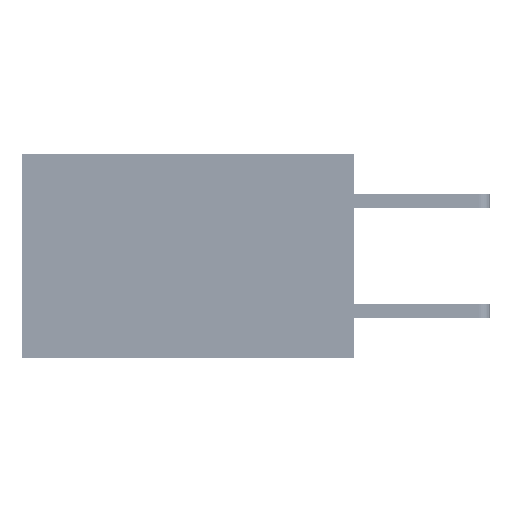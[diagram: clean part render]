
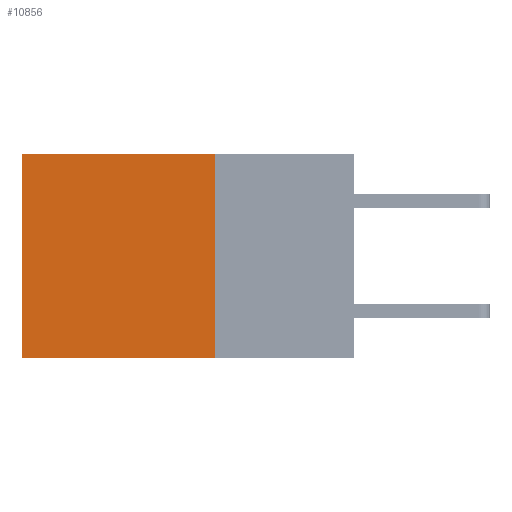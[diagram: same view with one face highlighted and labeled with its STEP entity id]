
A CAD part, left-side view. The second image highlights one B-rep face of the part: STEP entity #10856.
In plain terms, the highlighted planar face has unit normal (-1, 0, 0).
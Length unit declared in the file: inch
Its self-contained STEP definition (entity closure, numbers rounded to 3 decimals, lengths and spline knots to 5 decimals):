
#834 = EDGE_CURVE ( 'NONE', #1383, #25259, #34924, .T. ) ;
#1383 = VERTEX_POINT ( 'NONE', #32622 ) ;
#1986 = DIRECTION ( 'NONE',  ( 0., 1., 0. ) ) ;
#2571 = LINE ( 'NONE', #12450, #19545 ) ;
#5033 = VECTOR ( 'NONE', #1986, 39.37008 ) ;
#5194 = CARTESIAN_POINT ( 'NONE',  ( 0.2875, 0.6, -0.37 ) ) ;
#5345 = DIRECTION ( 'NONE',  ( 1., 0., 0. ) ) ;
#5413 = VERTEX_POINT ( 'NONE', #5194 ) ;
#10572 = EDGE_CURVE ( 'NONE', #1383, #33118, #15360, .T. ) ;
#10856 = ADVANCED_FACE ( 'NONE', ( #25638 ), #35568, .F. ) ;
#12450 = CARTESIAN_POINT ( 'NONE',  ( 0.2875, 0.25, -0.37 ) ) ;
#13830 = ORIENTED_EDGE ( 'NONE', *, *, #36696, .T. ) ;
#14040 = ORIENTED_EDGE ( 'NONE', *, *, #22499, .F. ) ;
#15360 = LINE ( 'NONE', #41514, #5033 ) ;
#18775 = DIRECTION ( 'NONE',  ( 0., 0., -1. ) ) ;
#19130 = CARTESIAN_POINT ( 'NONE',  ( 0.2875, 0.25, 0. ) ) ;
#19545 = VECTOR ( 'NONE', #22377, 39.37008 ) ;
#22377 = DIRECTION ( 'NONE',  ( 0., 1., 0. ) ) ;
#22499 = EDGE_CURVE ( 'NONE', #25259, #5413, #2571, .T. ) ;
#23221 = CARTESIAN_POINT ( 'NONE',  ( 0.2875, 0.25, -0.37 ) ) ;
#23643 = VECTOR ( 'NONE', #18775, 39.37008 ) ;
#24660 = VECTOR ( 'NONE', #38017, 39.37008 ) ;
#25259 = VERTEX_POINT ( 'NONE', #23221 ) ;
#25638 = FACE_OUTER_BOUND ( 'NONE', #25856, .T. ) ;
#25856 = EDGE_LOOP ( 'NONE', ( #13830, #14040, #37893, #31315 ) ) ;
#28336 = CARTESIAN_POINT ( 'NONE',  ( 0.2875, 0.6, 0. ) ) ;
#28402 = DIRECTION ( 'NONE',  ( 0., 0., -1. ) ) ;
#31315 = ORIENTED_EDGE ( 'NONE', *, *, #10572, .T. ) ;
#32457 = AXIS2_PLACEMENT_3D ( 'NONE', #19130, #5345, #28402 ) ;
#32622 = CARTESIAN_POINT ( 'NONE',  ( 0.2875, 0.25, 0. ) ) ;
#33118 = VERTEX_POINT ( 'NONE', #34392 ) ;
#34392 = CARTESIAN_POINT ( 'NONE',  ( 0.2875, 0.6, 0. ) ) ;
#34523 = CARTESIAN_POINT ( 'NONE',  ( 0.2875, 0.25, 0. ) ) ;
#34924 = LINE ( 'NONE', #34523, #24660 ) ;
#35568 = PLANE ( 'NONE',  #32457 ) ;
#36696 = EDGE_CURVE ( 'NONE', #33118, #5413, #40151, .T. ) ;
#37893 = ORIENTED_EDGE ( 'NONE', *, *, #834, .F. ) ;
#38017 = DIRECTION ( 'NONE',  ( 0., 0., -1. ) ) ;
#40151 = LINE ( 'NONE', #28336, #23643 ) ;
#41514 = CARTESIAN_POINT ( 'NONE',  ( 0.2875, 0.25, 0. ) ) ;
